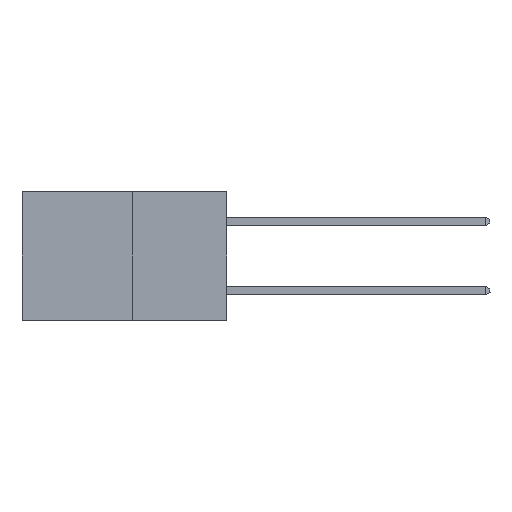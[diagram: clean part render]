
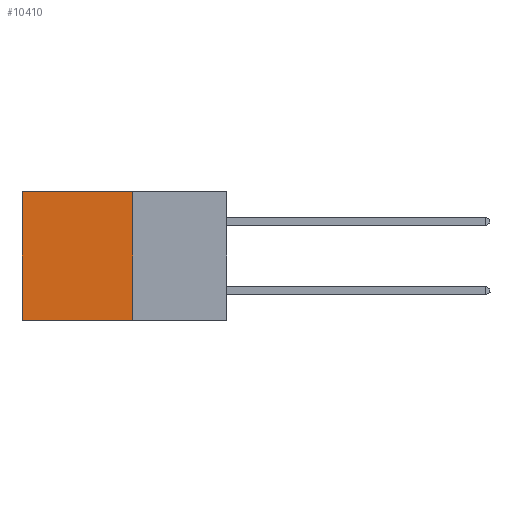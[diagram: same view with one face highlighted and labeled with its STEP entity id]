
A CAD part, left-side view. The second image highlights one B-rep face of the part: STEP entity #10410.
In plain terms, the highlighted planar face has unit normal (-1, 0, 0).
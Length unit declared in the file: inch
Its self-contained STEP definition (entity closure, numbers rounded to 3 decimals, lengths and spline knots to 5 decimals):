
#3 = CARTESIAN_POINT ( 'NONE',  ( 0.277, 0.27, -0.37 ) ) ;
#943 = DIRECTION ( 'NONE',  ( 0., 1., 0. ) ) ;
#975 = ORIENTED_EDGE ( 'NONE', *, *, #13853, .T. ) ;
#1256 = DIRECTION ( 'NONE',  ( 1., 0., 0. ) ) ;
#1650 = EDGE_CURVE ( 'NONE', #13648, #15412, #4645, .T. ) ;
#2688 = EDGE_CURVE ( 'NONE', #15473, #6376, #12412, .T. ) ;
#3510 = FACE_OUTER_BOUND ( 'NONE', #8529, .T. ) ;
#4645 = LINE ( 'NONE', #10542, #11127 ) ;
#5307 = CARTESIAN_POINT ( 'NONE',  ( 0.277, 0.27, -0.37 ) ) ;
#5353 = DIRECTION ( 'NONE',  ( 0., 1., 0. ) ) ;
#5834 = ORIENTED_EDGE ( 'NONE', *, *, #1650, .T. ) ;
#6173 = PLANE ( 'NONE',  #8438 ) ;
#6360 = EDGE_CURVE ( 'NONE', #13648, #15473, #6540, .T. ) ;
#6376 = VERTEX_POINT ( 'NONE', #7652 ) ;
#6397 = VECTOR ( 'NONE', #14313, 39.37008 ) ;
#6540 = LINE ( 'NONE', #7710, #12600 ) ;
#7126 = CARTESIAN_POINT ( 'NONE',  ( 0.277, 0.27, -0.37 ) ) ;
#7652 = CARTESIAN_POINT ( 'NONE',  ( 0.277, 0.59, -0.37 ) ) ;
#7691 = DIRECTION ( 'NONE',  ( 0., 0., -1. ) ) ;
#7710 = CARTESIAN_POINT ( 'NONE',  ( 0.277, 0.27, -0.37 ) ) ;
#8438 = AXIS2_PLACEMENT_3D ( 'NONE', #3, #1256, #9848 ) ;
#8529 = EDGE_LOOP ( 'NONE', ( #975, #10195, #15247, #5834 ) ) ;
#8837 = VECTOR ( 'NONE', #5353, 39.37008 ) ;
#9516 = CARTESIAN_POINT ( 'NONE',  ( 0.277, 0.59, -0.37 ) ) ;
#9650 = LINE ( 'NONE', #9516, #6397 ) ;
#9848 = DIRECTION ( 'NONE',  ( 0., 0., -1. ) ) ;
#10195 = ORIENTED_EDGE ( 'NONE', *, *, #2688, .F. ) ;
#10296 = CARTESIAN_POINT ( 'NONE',  ( 0.277, 0.27, 0. ) ) ;
#10410 = ADVANCED_FACE ( 'NONE', ( #3510 ), #6173, .F. ) ;
#10542 = CARTESIAN_POINT ( 'NONE',  ( 0.277, 0.27, 0. ) ) ;
#11127 = VECTOR ( 'NONE', #943, 39.37008 ) ;
#12412 = LINE ( 'NONE', #7126, #8837 ) ;
#12463 = CARTESIAN_POINT ( 'NONE',  ( 0.277, 0.59, 0. ) ) ;
#12600 = VECTOR ( 'NONE', #7691, 39.37008 ) ;
#13648 = VERTEX_POINT ( 'NONE', #10296 ) ;
#13853 = EDGE_CURVE ( 'NONE', #15412, #6376, #9650, .T. ) ;
#14313 = DIRECTION ( 'NONE',  ( 0., 0., -1. ) ) ;
#15247 = ORIENTED_EDGE ( 'NONE', *, *, #6360, .F. ) ;
#15412 = VERTEX_POINT ( 'NONE', #12463 ) ;
#15473 = VERTEX_POINT ( 'NONE', #5307 ) ;
